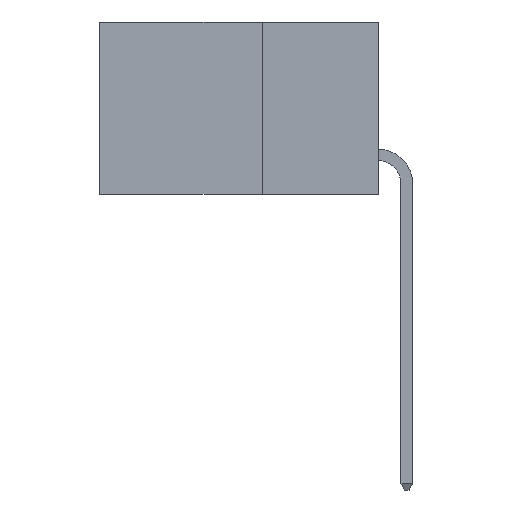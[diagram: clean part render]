
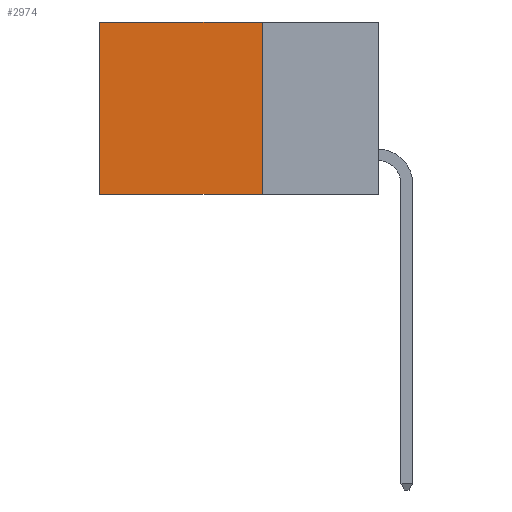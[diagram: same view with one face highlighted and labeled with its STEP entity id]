
A CAD part, left-side view. The second image highlights one B-rep face of the part: STEP entity #2974.
In plain terms, the highlighted planar face has unit normal (-1, 0, 0).
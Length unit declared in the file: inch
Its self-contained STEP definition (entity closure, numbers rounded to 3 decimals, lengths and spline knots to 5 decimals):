
#53 = EDGE_CURVE ( 'NONE', #1242, #2803, #4640, .T. ) ;
#178 = DIRECTION ( 'NONE',  ( 0., 0., -1. ) ) ;
#471 = LINE ( 'NONE', #4990, #2104 ) ;
#721 = FACE_OUTER_BOUND ( 'NONE', #5981, .T. ) ;
#842 = CARTESIAN_POINT ( 'NONE',  ( 0.2615, 0.25, -0.37 ) ) ;
#956 = ORIENTED_EDGE ( 'NONE', *, *, #1705, .T. ) ;
#982 = VECTOR ( 'NONE', #4871, 39.37008 ) ;
#1204 = AXIS2_PLACEMENT_3D ( 'NONE', #1921, #5510, #5795 ) ;
#1242 = VERTEX_POINT ( 'NONE', #5888 ) ;
#1514 = LINE ( 'NONE', #6227, #2946 ) ;
#1556 = EDGE_CURVE ( 'NONE', #6402, #1242, #7335, .T. ) ;
#1705 = EDGE_CURVE ( 'NONE', #6402, #5229, #1514, .T. ) ;
#1921 = CARTESIAN_POINT ( 'NONE',  ( 0.2615, 0.25, -0.37 ) ) ;
#2104 = VECTOR ( 'NONE', #178, 39.37008 ) ;
#2170 = VECTOR ( 'NONE', #4304, 39.37008 ) ;
#2407 = PLANE ( 'NONE',  #1204 ) ;
#2607 = CARTESIAN_POINT ( 'NONE',  ( 0.2615, 0.6, -0.37 ) ) ;
#2803 = VERTEX_POINT ( 'NONE', #2607 ) ;
#2946 = VECTOR ( 'NONE', #6616, 39.37008 ) ;
#2974 = ADVANCED_FACE ( 'NONE', ( #721 ), #2407, .F. ) ;
#3326 = CARTESIAN_POINT ( 'NONE',  ( 0.2615, 0.25, 0. ) ) ;
#4198 = ORIENTED_EDGE ( 'NONE', *, *, #53, .F. ) ;
#4304 = DIRECTION ( 'NONE',  ( 0., 0., -1. ) ) ;
#4640 = LINE ( 'NONE', #842, #982 ) ;
#4871 = DIRECTION ( 'NONE',  ( 0., 1., 0. ) ) ;
#4990 = CARTESIAN_POINT ( 'NONE',  ( 0.2615, 0.6, -0.37 ) ) ;
#5229 = VERTEX_POINT ( 'NONE', #5931 ) ;
#5322 = CARTESIAN_POINT ( 'NONE',  ( 0.2615, 0.25, -0.37 ) ) ;
#5510 = DIRECTION ( 'NONE',  ( 1., 0., 0. ) ) ;
#5511 = EDGE_CURVE ( 'NONE', #5229, #2803, #471, .T. ) ;
#5528 = ORIENTED_EDGE ( 'NONE', *, *, #5511, .T. ) ;
#5795 = DIRECTION ( 'NONE',  ( 0., 0., -1. ) ) ;
#5888 = CARTESIAN_POINT ( 'NONE',  ( 0.2615, 0.25, -0.37 ) ) ;
#5931 = CARTESIAN_POINT ( 'NONE',  ( 0.2615, 0.6, 0. ) ) ;
#5981 = EDGE_LOOP ( 'NONE', ( #5528, #4198, #6102, #956 ) ) ;
#6102 = ORIENTED_EDGE ( 'NONE', *, *, #1556, .F. ) ;
#6227 = CARTESIAN_POINT ( 'NONE',  ( 0.2615, 0.25, 0. ) ) ;
#6402 = VERTEX_POINT ( 'NONE', #3326 ) ;
#6616 = DIRECTION ( 'NONE',  ( 0., 1., 0. ) ) ;
#7335 = LINE ( 'NONE', #5322, #2170 ) ;
